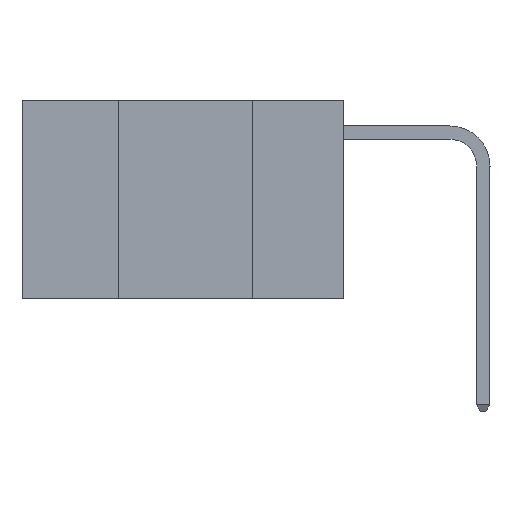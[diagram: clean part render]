
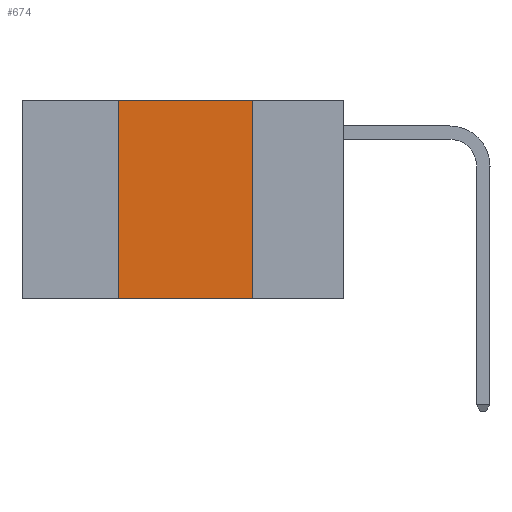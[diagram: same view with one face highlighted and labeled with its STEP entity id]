
A CAD part, left-side view. The second image highlights one B-rep face of the part: STEP entity #674.
In plain terms, the highlighted planar face has unit normal (-1, 0, 0).
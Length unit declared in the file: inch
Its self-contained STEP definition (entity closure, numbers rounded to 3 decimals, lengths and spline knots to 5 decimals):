
#24 = CARTESIAN_POINT ( 'NONE',  ( 0., 0.6, 0. ) ) ;
#120 = VERTEX_POINT ( 'NONE', #11067 ) ;
#267 = LINE ( 'NONE', #10141, #7068 ) ;
#520 = DIRECTION ( 'NONE',  ( 1., 0., 0. ) ) ;
#577 = EDGE_CURVE ( 'NONE', #1436, #120, #7570, .T. ) ;
#674 = ADVANCED_FACE ( 'NONE', ( #1806 ), #6553, .F. ) ;
#744 = VERTEX_POINT ( 'NONE', #3711 ) ;
#1436 = VERTEX_POINT ( 'NONE', #11076 ) ;
#1806 = FACE_OUTER_BOUND ( 'NONE', #3865, .T. ) ;
#1811 = DIRECTION ( 'NONE',  ( 0., 0., -1. ) ) ;
#2585 = EDGE_CURVE ( 'NONE', #2626, #1436, #7258, .T. ) ;
#2600 = CARTESIAN_POINT ( 'NONE',  ( 0., 0.42, 0. ) ) ;
#2626 = VERTEX_POINT ( 'NONE', #10322 ) ;
#3461 = VECTOR ( 'NONE', #4790, 39.37008 ) ;
#3711 = CARTESIAN_POINT ( 'NONE',  ( 0., 0.17, -0.37 ) ) ;
#3865 = EDGE_LOOP ( 'NONE', ( #10486, #4290, #4409, #7750 ) ) ;
#4229 = DIRECTION ( 'NONE',  ( 0., -1., 0. ) ) ;
#4290 = ORIENTED_EDGE ( 'NONE', *, *, #577, .F. ) ;
#4382 = DIRECTION ( 'NONE',  ( 0., 0., 1. ) ) ;
#4409 = ORIENTED_EDGE ( 'NONE', *, *, #2585, .F. ) ;
#4790 = DIRECTION ( 'NONE',  ( 0., 0., -1. ) ) ;
#5240 = EDGE_CURVE ( 'NONE', #2626, #744, #267, .T. ) ;
#5375 = AXIS2_PLACEMENT_3D ( 'NONE', #8639, #520, #1811 ) ;
#5506 = LINE ( 'NONE', #10673, #3461 ) ;
#5513 = DIRECTION ( 'NONE',  ( 0., -1., 0. ) ) ;
#6553 = PLANE ( 'NONE',  #5375 ) ;
#6703 = VECTOR ( 'NONE', #4382, 39.37008 ) ;
#7068 = VECTOR ( 'NONE', #4229, 39.37008 ) ;
#7258 = LINE ( 'NONE', #2600, #6703 ) ;
#7297 = VECTOR ( 'NONE', #5513, 39.37008 ) ;
#7570 = LINE ( 'NONE', #24, #7297 ) ;
#7750 = ORIENTED_EDGE ( 'NONE', *, *, #5240, .T. ) ;
#8639 = CARTESIAN_POINT ( 'NONE',  ( 0., 0.6, 0. ) ) ;
#9526 = EDGE_CURVE ( 'NONE', #120, #744, #5506, .T. ) ;
#10141 = CARTESIAN_POINT ( 'NONE',  ( 0., 0.6, -0.37 ) ) ;
#10322 = CARTESIAN_POINT ( 'NONE',  ( 0., 0.42, -0.37 ) ) ;
#10486 = ORIENTED_EDGE ( 'NONE', *, *, #9526, .F. ) ;
#10673 = CARTESIAN_POINT ( 'NONE',  ( 0., 0.17, 0. ) ) ;
#11067 = CARTESIAN_POINT ( 'NONE',  ( 0., 0.17, 0. ) ) ;
#11076 = CARTESIAN_POINT ( 'NONE',  ( 0., 0.42, 0. ) ) ;
